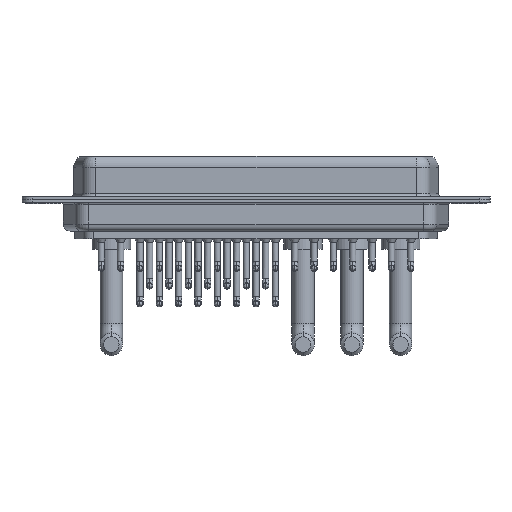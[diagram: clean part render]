
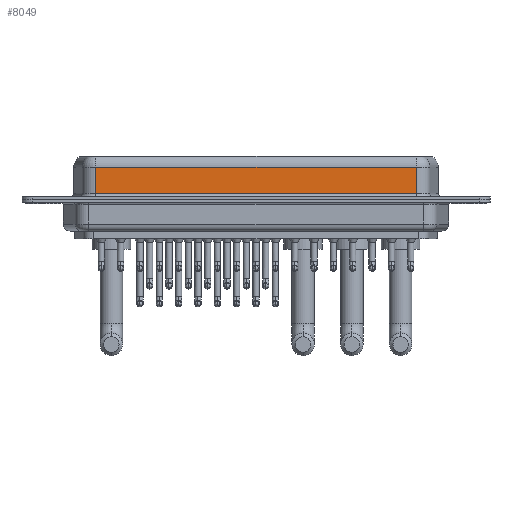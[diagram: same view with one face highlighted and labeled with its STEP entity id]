
A CAD part, front view. The second image highlights one B-rep face of the part: STEP entity #8049.
In plain terms, the highlighted planar face has unit normal (0, -1, 0).
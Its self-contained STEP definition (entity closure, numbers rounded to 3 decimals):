
#1807 = VERTEX_POINT ( 'NONE', #17089 ) ;
#2722 = ORIENTED_EDGE ( 'NONE', *, *, #25894, .T. ) ;
#3463 = EDGE_CURVE ( 'NONE', #4152, #23290, #12208, .T. ) ;
#3991 = EDGE_CURVE ( 'NONE', #4152, #1807, #7879, .T. ) ;
#4152 = VERTEX_POINT ( 'NONE', #13402 ) ;
#5223 = ORIENTED_EDGE ( 'NONE', *, *, #3991, .T. ) ;
#7879 = LINE ( 'NONE', #22925, #12875 ) ;
#8049 = ADVANCED_FACE ( 'NONE', ( #18074 ), #13597, .F. ) ;
#8672 = ORIENTED_EDGE ( 'NONE', *, *, #13990, .T. ) ;
#9704 = VECTOR ( 'NONE', #27281, 1000. ) ;
#11908 = VECTOR ( 'NONE', #20867, 1000. ) ;
#12057 = CARTESIAN_POINT ( 'NONE',  ( 53.41, -5.375, 6.4 ) ) ;
#12208 = LINE ( 'NONE', #20721, #9704 ) ;
#12211 = LINE ( 'NONE', #27284, #11908 ) ;
#12367 = EDGE_LOOP ( 'NONE', ( #27391, #5223, #8672, #2722 ) ) ;
#12875 = VECTOR ( 'NONE', #22791, 1000. ) ;
#13402 = CARTESIAN_POINT ( 'NONE',  ( 53.41, -5.375, 4.65 ) ) ;
#13597 = PLANE ( 'NONE',  #20577 ) ;
#13990 = EDGE_CURVE ( 'NONE', #1807, #15817, #12211, .T. ) ;
#14114 = CARTESIAN_POINT ( 'NONE',  ( 53.41, -5.375, 0.9 ) ) ;
#14156 = LINE ( 'NONE', #20441, #14190 ) ;
#14190 = VECTOR ( 'NONE', #26748, 1000. ) ;
#15817 = VERTEX_POINT ( 'NONE', #21885 ) ;
#17089 = CARTESIAN_POINT ( 'NONE',  ( 7.59, -5.375, 4.65 ) ) ;
#17797 = DIRECTION ( 'NONE',  ( 0., 0., 1. ) ) ;
#18074 = FACE_OUTER_BOUND ( 'NONE', #12367, .T. ) ;
#20441 = CARTESIAN_POINT ( 'NONE',  ( 53.41, -5.375, 0.9 ) ) ;
#20571 = DIRECTION ( 'NONE',  ( 0., 1., 0. ) ) ;
#20577 = AXIS2_PLACEMENT_3D ( 'NONE', #12057, #20571, #17797 ) ;
#20721 = CARTESIAN_POINT ( 'NONE',  ( 53.41, -5.375, 6.4 ) ) ;
#20867 = DIRECTION ( 'NONE',  ( 0., 0., -1. ) ) ;
#21885 = CARTESIAN_POINT ( 'NONE',  ( 7.59, -5.375, 0.9 ) ) ;
#22791 = DIRECTION ( 'NONE',  ( -1., 0., 0. ) ) ;
#22925 = CARTESIAN_POINT ( 'NONE',  ( 53.41, -5.375, 4.65 ) ) ;
#23290 = VERTEX_POINT ( 'NONE', #14114 ) ;
#25894 = EDGE_CURVE ( 'NONE', #15817, #23290, #14156, .T. ) ;
#26748 = DIRECTION ( 'NONE',  ( 1., 0., 0. ) ) ;
#27281 = DIRECTION ( 'NONE',  ( 0., 0., -1. ) ) ;
#27284 = CARTESIAN_POINT ( 'NONE',  ( 7.59, -5.375, 6.4 ) ) ;
#27391 = ORIENTED_EDGE ( 'NONE', *, *, #3463, .F. ) ;
